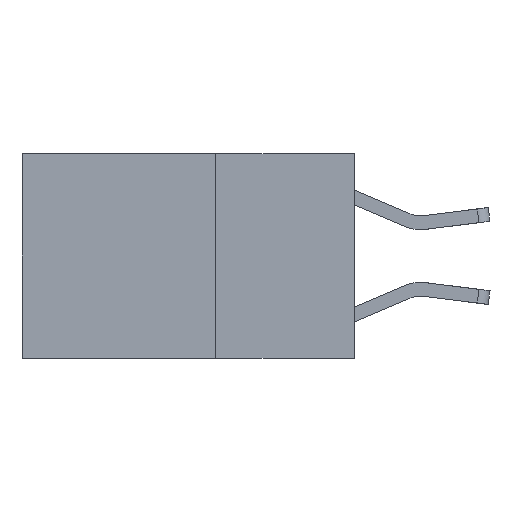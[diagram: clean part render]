
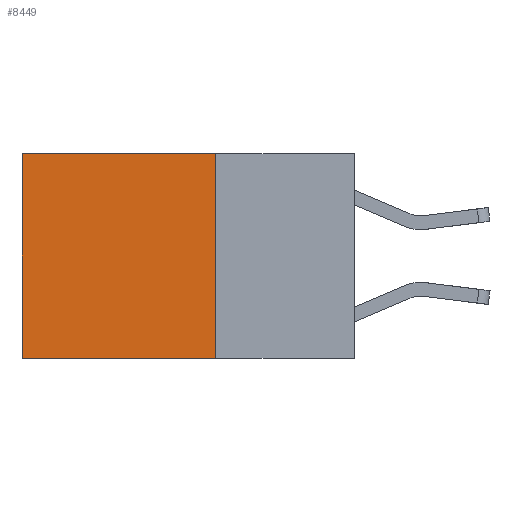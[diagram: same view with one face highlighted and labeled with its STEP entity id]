
A CAD part, left-side view. The second image highlights one B-rep face of the part: STEP entity #8449.
In plain terms, the highlighted planar face has unit normal (-1, 0, 0).
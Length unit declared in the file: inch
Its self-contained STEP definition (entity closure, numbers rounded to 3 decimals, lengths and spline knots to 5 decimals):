
#32 = VERTEX_POINT ( 'NONE', #4184 ) ;
#85 = LINE ( 'NONE', #921, #4317 ) ;
#498 = PLANE ( 'NONE',  #10831 ) ;
#921 = CARTESIAN_POINT ( 'NONE',  ( 0.2625, 0.25, 0. ) ) ;
#1256 = CARTESIAN_POINT ( 'NONE',  ( 0.2625, 0.25, -0.37 ) ) ;
#2086 = VECTOR ( 'NONE', #10208, 39.37008 ) ;
#2260 = CARTESIAN_POINT ( 'NONE',  ( 0.2625, 0.25, 0. ) ) ;
#2963 = VERTEX_POINT ( 'NONE', #6438 ) ;
#3062 = DIRECTION ( 'NONE',  ( 0., 0., -1. ) ) ;
#3396 = VERTEX_POINT ( 'NONE', #7551 ) ;
#3839 = VECTOR ( 'NONE', #5390, 39.37008 ) ;
#3915 = EDGE_CURVE ( 'NONE', #32, #4052, #8925, .T. ) ;
#4032 = CARTESIAN_POINT ( 'NONE',  ( 0.2625, 0.6, 0. ) ) ;
#4033 = DIRECTION ( 'NONE',  ( 0., 1., 0. ) ) ;
#4052 = VERTEX_POINT ( 'NONE', #6418 ) ;
#4184 = CARTESIAN_POINT ( 'NONE',  ( 0.2625, 0.25, -0.37 ) ) ;
#4283 = DIRECTION ( 'NONE',  ( 0., 0., -1. ) ) ;
#4317 = VECTOR ( 'NONE', #4283, 39.37008 ) ;
#5390 = DIRECTION ( 'NONE',  ( 0., 1., 0. ) ) ;
#5895 = ORIENTED_EDGE ( 'NONE', *, *, #3915, .F. ) ;
#5974 = ORIENTED_EDGE ( 'NONE', *, *, #7992, .F. ) ;
#6418 = CARTESIAN_POINT ( 'NONE',  ( 0.2625, 0.6, -0.37 ) ) ;
#6438 = CARTESIAN_POINT ( 'NONE',  ( 0.2625, 0.6, 0. ) ) ;
#6498 = LINE ( 'NONE', #10209, #10903 ) ;
#7551 = CARTESIAN_POINT ( 'NONE',  ( 0.2625, 0.25, 0. ) ) ;
#7710 = ORIENTED_EDGE ( 'NONE', *, *, #9301, .T. ) ;
#7902 = EDGE_CURVE ( 'NONE', #3396, #2963, #6498, .T. ) ;
#7992 = EDGE_CURVE ( 'NONE', #3396, #32, #85, .T. ) ;
#8434 = DIRECTION ( 'NONE',  ( 1., 0., 0. ) ) ;
#8449 = ADVANCED_FACE ( 'NONE', ( #9749 ), #498, .F. ) ;
#8925 = LINE ( 'NONE', #1256, #3839 ) ;
#9081 = LINE ( 'NONE', #4032, #2086 ) ;
#9141 = EDGE_LOOP ( 'NONE', ( #7710, #5895, #5974, #9795 ) ) ;
#9301 = EDGE_CURVE ( 'NONE', #2963, #4052, #9081, .T. ) ;
#9749 = FACE_OUTER_BOUND ( 'NONE', #9141, .T. ) ;
#9795 = ORIENTED_EDGE ( 'NONE', *, *, #7902, .T. ) ;
#10208 = DIRECTION ( 'NONE',  ( 0., 0., -1. ) ) ;
#10209 = CARTESIAN_POINT ( 'NONE',  ( 0.2625, 0.25, 0. ) ) ;
#10831 = AXIS2_PLACEMENT_3D ( 'NONE', #2260, #8434, #3062 ) ;
#10903 = VECTOR ( 'NONE', #4033, 39.37008 ) ;
